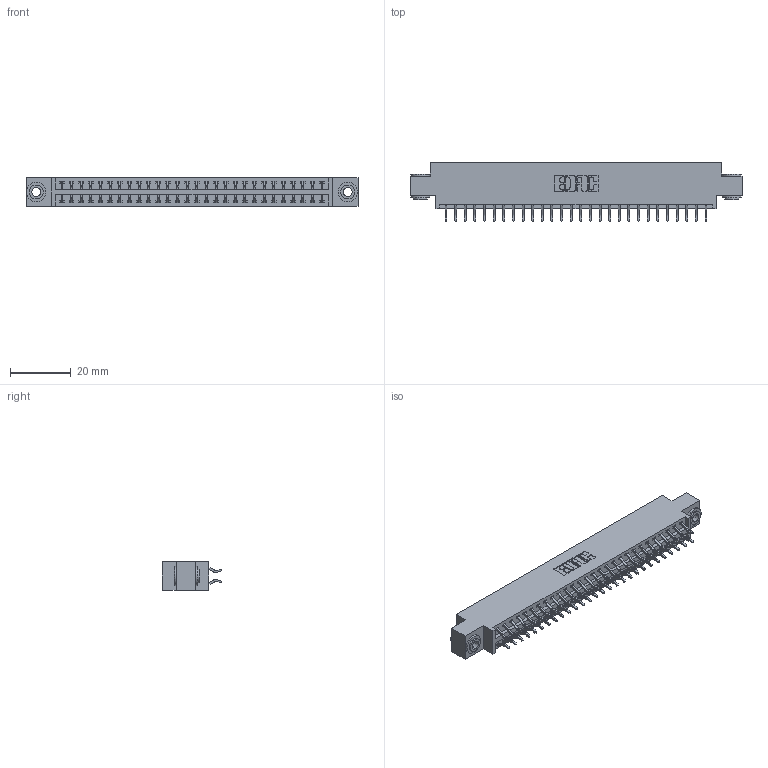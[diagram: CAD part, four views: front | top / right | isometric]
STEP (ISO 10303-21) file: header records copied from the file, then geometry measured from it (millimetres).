
FILE_DESCRIPTION (( 'STEP AP203' ), '1' );
FILE_NAME ('346-056-556-803.STEP', '2018-08-28T03:07:22', ( '' ), ( '' ), 'SwSTEP 2.0', 'SolidWorks 2016', '' );
FILE_SCHEMA (( 'CONFIG_CONTROL_DESIGN' ));
Length unit declared in the file: inch
Products named in the file (4): 346 Part_0.170 Offset - 0.156 Dia-TH; 345-292-001_556 Tail; 345-250-002_345-250-002-102; 346-056-556-803
Assembly tree (59 placements, depth 2):
  346-056-556-803
    346 Part_0.170 Offset - 0.156 Dia-TH
    345-292-001_556 Tail  x56
    345-250-002_345-250-002-102  x2
Bounding box: 109.47 x 19.57 x 9.4 mm (x, y, z)
Volume: 10428.9 mm3; surface area: 14457 mm2
Topology: 59 solids, 59 shells, 3412 faces, 10105 edges, 6658 vertices
Faces by surface type: plane 2274, cylinder 1130, cone 8
Entity records: 21160 total; most frequent: CARTESIAN_POINT 3499, ORIENTED_EDGE 3414, DIRECTION 3153, EDGE_CURVE 1707, VECTOR 1431, LINE 1431, VERTEX_POINT 1134, AXIS2_PLACEMENT_3D 861
